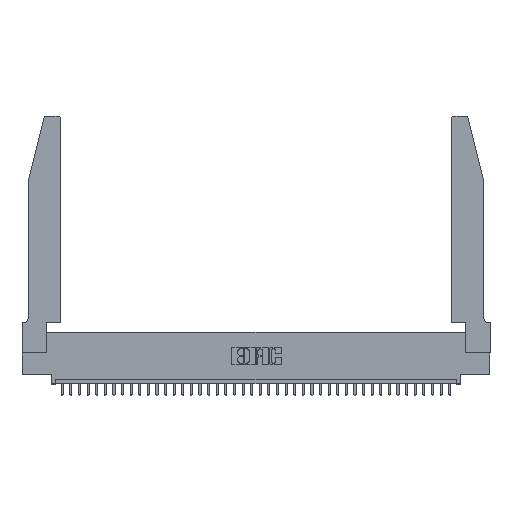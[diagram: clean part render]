
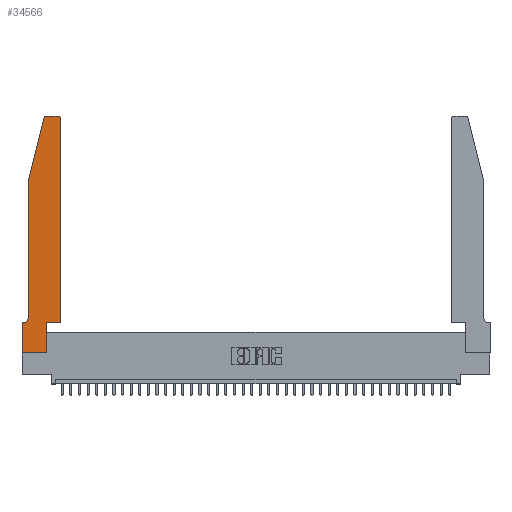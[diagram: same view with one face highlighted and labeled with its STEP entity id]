
A CAD part, top view. The second image highlights one B-rep face of the part: STEP entity #34566.
In plain terms, the highlighted planar face has unit normal (0, 0, 1).
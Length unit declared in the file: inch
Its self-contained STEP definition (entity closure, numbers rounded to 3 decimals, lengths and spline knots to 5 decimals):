
#467 = VERTEX_POINT ( 'NONE', #5356 ) ;
#494 = DIRECTION ( 'NONE',  ( 1., 0., 0. ) ) ;
#912 = ORIENTED_EDGE ( 'NONE', *, *, #27328, .T. ) ;
#1036 = CARTESIAN_POINT ( 'NONE',  ( 0.0755, 0.35, 0.37 ) ) ;
#1542 = VERTEX_POINT ( 'NONE', #24261 ) ;
#1641 = VECTOR ( 'NONE', #5409, 39.37008 ) ;
#1954 = CIRCLE ( 'NONE', #8674, 0.07 ) ;
#3001 = DIRECTION ( 'NONE',  ( 0., 0., -1. ) ) ;
#4370 = LINE ( 'NONE', #30591, #15149 ) ;
#4790 = EDGE_CURVE ( 'NONE', #11220, #23980, #20594, .T. ) ;
#5147 = VERTEX_POINT ( 'NONE', #9739 ) ;
#5267 = ORIENTED_EDGE ( 'NONE', *, *, #32231, .T. ) ;
#5356 = CARTESIAN_POINT ( 'NONE',  ( 0.2865, 0., 0.37 ) ) ;
#5409 = DIRECTION ( 'NONE',  ( 0., -1., 0. ) ) ;
#5789 = VECTOR ( 'NONE', #494, 39.37008 ) ;
#5875 = VECTOR ( 'NONE', #9411, 39.37008 ) ;
#6129 = VECTOR ( 'NONE', #31745, 39.37008 ) ;
#6963 = VERTEX_POINT ( 'NONE', #28391 ) ;
#8078 = LINE ( 'NONE', #36757, #11337 ) ;
#8111 = CARTESIAN_POINT ( 'NONE',  ( 0.0055, 0.42, 0.37 ) ) ;
#8674 = AXIS2_PLACEMENT_3D ( 'NONE', #8111, #3001, #38823 ) ;
#8675 = CARTESIAN_POINT ( 'NONE',  ( 0., 0., 0.37 ) ) ;
#9115 = DIRECTION ( 'NONE',  ( 1., 0., 0. ) ) ;
#9245 = ORIENTED_EDGE ( 'NONE', *, *, #36494, .T. ) ;
#9319 = CARTESIAN_POINT ( 'NONE',  ( 0., 0., 0.37 ) ) ;
#9411 = DIRECTION ( 'NONE',  ( 1., 0., 0. ) ) ;
#9726 = EDGE_CURVE ( 'NONE', #1542, #35295, #16954, .T. ) ;
#9739 = CARTESIAN_POINT ( 'NONE',  ( 0.0055, 0.35, 0.37 ) ) ;
#10074 = LINE ( 'NONE', #8675, #1641 ) ;
#10232 = CARTESIAN_POINT ( 'NONE',  ( 0.4505, 0.35, 0.37 ) ) ;
#10687 = CARTESIAN_POINT ( 'NONE',  ( 0.2865, 0.35, 0.37 ) ) ;
#11220 = VERTEX_POINT ( 'NONE', #11911 ) ;
#11337 = VECTOR ( 'NONE', #27670, 39.37008 ) ;
#11579 = CARTESIAN_POINT ( 'NONE',  ( 0., 0.35, 0.37 ) ) ;
#11699 = CARTESIAN_POINT ( 'NONE',  ( 0., 0.35, 0.37 ) ) ;
#11911 = CARTESIAN_POINT ( 'NONE',  ( 0.4505, 2.72, 0.37 ) ) ;
#12385 = LINE ( 'NONE', #29309, #5875 ) ;
#12883 = DIRECTION ( 'NONE',  ( -0.239, -0.971, 0. ) ) ;
#12978 = DIRECTION ( 'NONE',  ( 1., 0., 0. ) ) ;
#13636 = VERTEX_POINT ( 'NONE', #10687 ) ;
#13916 = AXIS2_PLACEMENT_3D ( 'NONE', #11579, #35825, #20785 ) ;
#14039 = AXIS2_PLACEMENT_3D ( 'NONE', #29004, #36955, #12978 ) ;
#14049 = ORIENTED_EDGE ( 'NONE', *, *, #29644, .T. ) ;
#15149 = VECTOR ( 'NONE', #15314, 39.37008 ) ;
#15314 = DIRECTION ( 'NONE',  ( -1., 0., 0. ) ) ;
#15969 = DIRECTION ( 'NONE',  ( 0., 1., 0. ) ) ;
#16281 = ORIENTED_EDGE ( 'NONE', *, *, #20651, .T. ) ;
#16912 = LINE ( 'NONE', #38130, #26832 ) ;
#16954 = LINE ( 'NONE', #28052, #25443 ) ;
#18185 = ORIENTED_EDGE ( 'NONE', *, *, #9726, .T. ) ;
#18846 = ORIENTED_EDGE ( 'NONE', *, *, #38505, .T. ) ;
#19270 = ORIENTED_EDGE ( 'NONE', *, *, #32125, .T. ) ;
#19847 = VERTEX_POINT ( 'NONE', #11699 ) ;
#20083 = FACE_OUTER_BOUND ( 'NONE', #35352, .T. ) ;
#20130 = AXIS2_PLACEMENT_3D ( 'NONE', #33064, #34293, #9115 ) ;
#20594 = CIRCLE ( 'NONE', #14039, 0.03 ) ;
#20651 = EDGE_CURVE ( 'NONE', #13636, #21762, #12385, .T. ) ;
#20785 = DIRECTION ( 'NONE',  ( 1., 0., 0. ) ) ;
#20834 = ORIENTED_EDGE ( 'NONE', *, *, #32539, .T. ) ;
#21256 = CARTESIAN_POINT ( 'NONE',  ( 0., 0., 0.37 ) ) ;
#21762 = VERTEX_POINT ( 'NONE', #10232 ) ;
#22120 = LINE ( 'NONE', #31199, #6129 ) ;
#22329 = CARTESIAN_POINT ( 'NONE',  ( 0.4205, 2.75, 0.37 ) ) ;
#22638 = EDGE_CURVE ( 'NONE', #5147, #19847, #38775, .T. ) ;
#23980 = VERTEX_POINT ( 'NONE', #22329 ) ;
#24143 = CARTESIAN_POINT ( 'NONE',  ( 0.0755, 2., 0.37 ) ) ;
#24261 = CARTESIAN_POINT ( 'NONE',  ( 0.25487, 2.72718, 0.37 ) ) ;
#24464 = ORIENTED_EDGE ( 'NONE', *, *, #22638, .T. ) ;
#24874 = ORIENTED_EDGE ( 'NONE', *, *, #36548, .T. ) ;
#25443 = VECTOR ( 'NONE', #12883, 39.37008 ) ;
#26283 = DIRECTION ( 'NONE',  ( -1., 0., 0. ) ) ;
#26488 = VERTEX_POINT ( 'NONE', #9319 ) ;
#26832 = VECTOR ( 'NONE', #15969, 39.37008 ) ;
#27328 = EDGE_CURVE ( 'NONE', #467, #13636, #16912, .T. ) ;
#27670 = DIRECTION ( 'NONE',  ( 0., 1., 0. ) ) ;
#28052 = CARTESIAN_POINT ( 'NONE',  ( 0.0755, 2., 0.37 ) ) ;
#28391 = CARTESIAN_POINT ( 'NONE',  ( 0.284, 2.75, 0.37 ) ) ;
#29004 = CARTESIAN_POINT ( 'NONE',  ( 0.4205, 2.72, 0.37 ) ) ;
#29309 = CARTESIAN_POINT ( 'NONE',  ( 0.4505, 0.35, 0.37 ) ) ;
#29644 = EDGE_CURVE ( 'NONE', #19847, #26488, #10074, .T. ) ;
#30591 = CARTESIAN_POINT ( 'NONE',  ( 0.2605, 2.75, 0.37 ) ) ;
#30703 = LINE ( 'NONE', #21256, #5789 ) ;
#31199 = CARTESIAN_POINT ( 'NONE',  ( 0.0755, 2., 0.37 ) ) ;
#31745 = DIRECTION ( 'NONE',  ( 0., -1., 0. ) ) ;
#32125 = EDGE_CURVE ( 'NONE', #21762, #11220, #8078, .T. ) ;
#32231 = EDGE_CURVE ( 'NONE', #6963, #1542, #35864, .T. ) ;
#32539 = EDGE_CURVE ( 'NONE', #35295, #38268, #22120, .T. ) ;
#33064 = CARTESIAN_POINT ( 'NONE',  ( 0.284, 2.72, 0.37 ) ) ;
#34293 = DIRECTION ( 'NONE',  ( 0., 0., 1. ) ) ;
#34477 = CARTESIAN_POINT ( 'NONE',  ( 0.0755, 0.42, 0.37 ) ) ;
#34566 = ADVANCED_FACE ( 'NONE', ( #20083 ), #38751, .T. ) ;
#35295 = VERTEX_POINT ( 'NONE', #24143 ) ;
#35352 = EDGE_LOOP ( 'NONE', ( #24874, #5267, #18185, #20834, #18846, #24464, #14049, #9245, #912, #16281, #19270, #35636 ) ) ;
#35636 = ORIENTED_EDGE ( 'NONE', *, *, #4790, .T. ) ;
#35825 = DIRECTION ( 'NONE',  ( 0., 0., 1. ) ) ;
#35864 = CIRCLE ( 'NONE', #20130, 0.03 ) ;
#36494 = EDGE_CURVE ( 'NONE', #26488, #467, #30703, .T. ) ;
#36548 = EDGE_CURVE ( 'NONE', #23980, #6963, #4370, .T. ) ;
#36757 = CARTESIAN_POINT ( 'NONE',  ( 0.4505, 0.35, 0.37 ) ) ;
#36955 = DIRECTION ( 'NONE',  ( 0., 0., 1. ) ) ;
#37359 = VECTOR ( 'NONE', #26283, 39.37008 ) ;
#38130 = CARTESIAN_POINT ( 'NONE',  ( 0.2865, 0.35, 0.37 ) ) ;
#38268 = VERTEX_POINT ( 'NONE', #34477 ) ;
#38505 = EDGE_CURVE ( 'NONE', #38268, #5147, #1954, .T. ) ;
#38751 = PLANE ( 'NONE',  #13916 ) ;
#38775 = LINE ( 'NONE', #1036, #37359 ) ;
#38823 = DIRECTION ( 'NONE',  ( -1., 0., 0. ) ) ;
